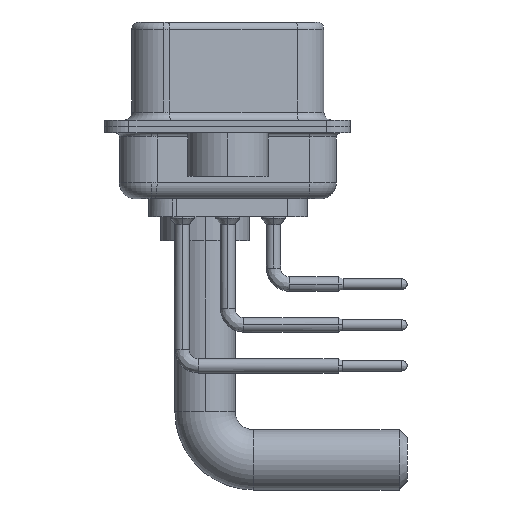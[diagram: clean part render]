
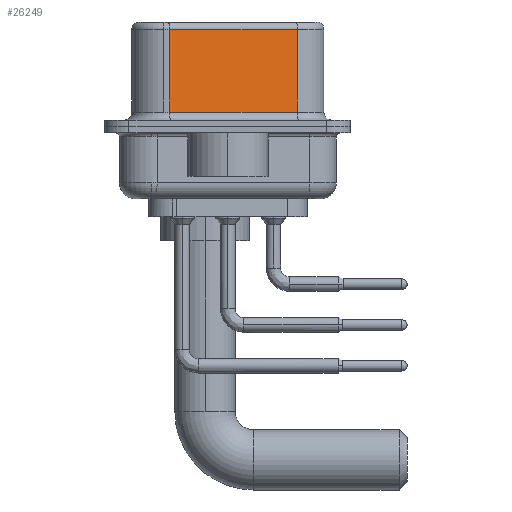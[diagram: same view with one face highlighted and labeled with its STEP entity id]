
A CAD part, left-side view. The second image highlights one B-rep face of the part: STEP entity #26249.
In plain terms, the highlighted planar face has unit normal (-0.985, -0.174, 0).
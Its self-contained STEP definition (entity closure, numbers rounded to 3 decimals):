
#409 = ORIENTED_EDGE ( 'NONE', *, *, #1041, .T. ) ;
#488 = LINE ( 'NONE', #23940, #29732 ) ;
#1041 = EDGE_CURVE ( 'NONE', #17442, #6793, #488, .T. ) ;
#1519 = LINE ( 'NONE', #33316, #30827 ) ;
#3359 = CARTESIAN_POINT ( 'NONE',  ( 5.132, -4.322, 6.52 ) ) ;
#4550 = EDGE_LOOP ( 'NONE', ( #34067, #409, #26726, #9814 ) ) ;
#4723 = DIRECTION ( 'NONE',  ( 0.174, -0.985, 0. ) ) ;
#6793 = VERTEX_POINT ( 'NONE', #16971 ) ;
#7329 = CARTESIAN_POINT ( 'NONE',  ( 3.73, 3.628, 6.52 ) ) ;
#9814 = ORIENTED_EDGE ( 'NONE', *, *, #10621, .T. ) ;
#10621 = EDGE_CURVE ( 'NONE', #24217, #30573, #1519, .T. ) ;
#14424 = CARTESIAN_POINT ( 'NONE',  ( 3.73, 3.628, 0.9 ) ) ;
#14537 = DIRECTION ( 'NONE',  ( 0., 0., -1. ) ) ;
#15510 = VECTOR ( 'NONE', #14537, 1000. ) ;
#16971 = CARTESIAN_POINT ( 'NONE',  ( 3.73, 3.628, 6.02 ) ) ;
#17442 = VERTEX_POINT ( 'NONE', #34780 ) ;
#19560 = VECTOR ( 'NONE', #30998, 1000. ) ;
#23940 = CARTESIAN_POINT ( 'NONE',  ( 5.132, -4.322, 6.02 ) ) ;
#24217 = VERTEX_POINT ( 'NONE', #14424 ) ;
#25291 = AXIS2_PLACEMENT_3D ( 'NONE', #30632, #30454, #33653 ) ;
#26249 = ADVANCED_FACE ( 'NONE', ( #27428 ), #35946, .F. ) ;
#26726 = ORIENTED_EDGE ( 'NONE', *, *, #32307, .T. ) ;
#27428 = FACE_OUTER_BOUND ( 'NONE', #4550, .T. ) ;
#27591 = CARTESIAN_POINT ( 'NONE',  ( 5.132, -4.322, 0.9 ) ) ;
#29732 = VECTOR ( 'NONE', #35512, 1000. ) ;
#30454 = DIRECTION ( 'NONE',  ( 0.985, 0.174, 0. ) ) ;
#30573 = VERTEX_POINT ( 'NONE', #27591 ) ;
#30611 = LINE ( 'NONE', #7329, #19560 ) ;
#30632 = CARTESIAN_POINT ( 'NONE',  ( 5.132, -4.322, 6.52 ) ) ;
#30827 = VECTOR ( 'NONE', #4723, 1000. ) ;
#30998 = DIRECTION ( 'NONE',  ( 0., 0., -1. ) ) ;
#32307 = EDGE_CURVE ( 'NONE', #6793, #24217, #30611, .T. ) ;
#32326 = LINE ( 'NONE', #3359, #15510 ) ;
#33316 = CARTESIAN_POINT ( 'NONE',  ( 5.132, -4.322, 0.9 ) ) ;
#33653 = DIRECTION ( 'NONE',  ( -0.174, 0.985, 0. ) ) ;
#34067 = ORIENTED_EDGE ( 'NONE', *, *, #35033, .F. ) ;
#34780 = CARTESIAN_POINT ( 'NONE',  ( 5.132, -4.322, 6.02 ) ) ;
#35033 = EDGE_CURVE ( 'NONE', #17442, #30573, #32326, .T. ) ;
#35512 = DIRECTION ( 'NONE',  ( -0.174, 0.985, 0. ) ) ;
#35946 = PLANE ( 'NONE',  #25291 ) ;
